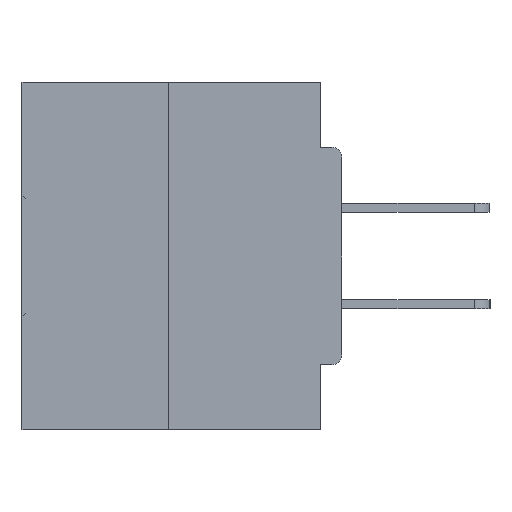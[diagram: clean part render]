
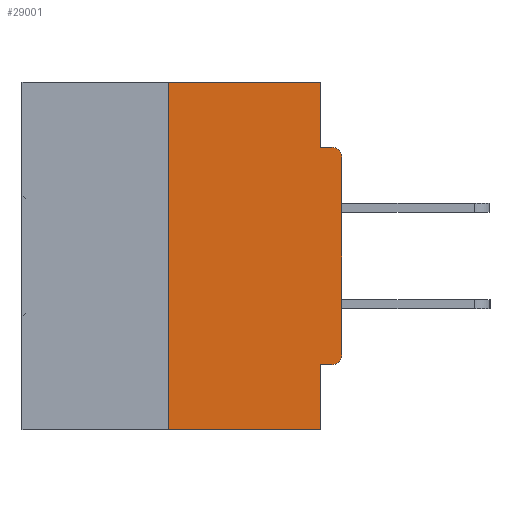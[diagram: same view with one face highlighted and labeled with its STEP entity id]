
A CAD part, left-side view. The second image highlights one B-rep face of the part: STEP entity #29001.
In plain terms, the highlighted planar face has unit normal (-1, 0, 0).
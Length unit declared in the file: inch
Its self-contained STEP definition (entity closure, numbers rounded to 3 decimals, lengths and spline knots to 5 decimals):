
#209 = CARTESIAN_POINT ( 'NONE',  ( 0., 0., -0.4065 ) ) ;
#803 = DIRECTION ( 'NONE',  ( 0., -1., 0. ) ) ;
#871 = VECTOR ( 'NONE', #2284, 39.37008 ) ;
#1094 = CARTESIAN_POINT ( 'NONE',  ( 0., 0.015, -0.4065 ) ) ;
#1310 = DIRECTION ( 'NONE',  ( 0., 0., -1. ) ) ;
#2025 = VERTEX_POINT ( 'NONE', #38893 ) ;
#2284 = DIRECTION ( 'NONE',  ( 0., 0., -1. ) ) ;
#2724 = DIRECTION ( 'NONE',  ( -1., 0., 0. ) ) ;
#3102 = CARTESIAN_POINT ( 'NONE',  ( 0., 0., -0.1085 ) ) ;
#3535 = CARTESIAN_POINT ( 'NONE',  ( 0., 0.25, 0. ) ) ;
#3756 = EDGE_CURVE ( 'NONE', #33073, #25806, #28553, .T. ) ;
#5375 = EDGE_CURVE ( 'NONE', #2025, #14541, #27541, .T. ) ;
#5636 = ORIENTED_EDGE ( 'NONE', *, *, #16228, .T. ) ;
#5768 = CARTESIAN_POINT ( 'NONE',  ( 0., 0.015, -0.3915 ) ) ;
#6494 = ORIENTED_EDGE ( 'NONE', *, *, #5375, .F. ) ;
#9302 = VECTOR ( 'NONE', #24509, 39.37008 ) ;
#9380 = ORIENTED_EDGE ( 'NONE', *, *, #10526, .T. ) ;
#9419 = VERTEX_POINT ( 'NONE', #3102 ) ;
#10275 = CARTESIAN_POINT ( 'NONE',  ( 0., 0.46, -0.5 ) ) ;
#10526 = EDGE_CURVE ( 'NONE', #12699, #25806, #32915, .T. ) ;
#11445 = EDGE_CURVE ( 'NONE', #33711, #33073, #29944, .T. ) ;
#12699 = VERTEX_POINT ( 'NONE', #19919 ) ;
#12700 = EDGE_LOOP ( 'NONE', ( #19458, #32668, #9380, #21353, #15758, #39496, #5636, #24989, #30597, #6494 ) ) ;
#12721 = VECTOR ( 'NONE', #803, 39.37008 ) ;
#14541 = VERTEX_POINT ( 'NONE', #25181 ) ;
#14918 = VECTOR ( 'NONE', #36881, 39.37008 ) ;
#15758 = ORIENTED_EDGE ( 'NONE', *, *, #11445, .F. ) ;
#15767 = DIRECTION ( 'NONE',  ( 0., -1., 0. ) ) ;
#16208 = LINE ( 'NONE', #32558, #35334 ) ;
#16228 = EDGE_CURVE ( 'NONE', #28653, #9419, #24288, .T. ) ;
#17284 = CARTESIAN_POINT ( 'NONE',  ( 0., 0., -0.0935 ) ) ;
#17497 = LINE ( 'NONE', #17284, #12721 ) ;
#19458 = ORIENTED_EDGE ( 'NONE', *, *, #29046, .F. ) ;
#19919 = CARTESIAN_POINT ( 'NONE',  ( 0., 0.25, -0.5 ) ) ;
#20221 = AXIS2_PLACEMENT_3D ( 'NONE', #5768, #28376, #38171 ) ;
#21062 = CARTESIAN_POINT ( 'NONE',  ( 0., 0.46, 0. ) ) ;
#21353 = ORIENTED_EDGE ( 'NONE', *, *, #3756, .F. ) ;
#22382 = CARTESIAN_POINT ( 'NONE',  ( 0., 0., -0.3915 ) ) ;
#23058 = CIRCLE ( 'NONE', #32781, 0.015 ) ;
#23526 = DIRECTION ( 'NONE',  ( 0., -1., 0. ) ) ;
#23852 = CARTESIAN_POINT ( 'NONE',  ( 0., 0.031, 0. ) ) ;
#24288 = LINE ( 'NONE', #31470, #37055 ) ;
#24320 = PLANE ( 'NONE',  #31164 ) ;
#24509 = DIRECTION ( 'NONE',  ( 0., 0., -1. ) ) ;
#24989 = ORIENTED_EDGE ( 'NONE', *, *, #27829, .T. ) ;
#25181 = CARTESIAN_POINT ( 'NONE',  ( 0., 0.031, -0.0935 ) ) ;
#25806 = VERTEX_POINT ( 'NONE', #35751 ) ;
#27541 = LINE ( 'NONE', #23852, #9302 ) ;
#27630 = EDGE_CURVE ( 'NONE', #33711, #28653, #35540, .T. ) ;
#27829 = EDGE_CURVE ( 'NONE', #9419, #33159, #23058, .T. ) ;
#28376 = DIRECTION ( 'NONE',  ( -1., 0., 0. ) ) ;
#28553 = LINE ( 'NONE', #38150, #871 ) ;
#28653 = VERTEX_POINT ( 'NONE', #22382 ) ;
#29001 = ADVANCED_FACE ( 'NONE', ( #40858 ), #24320, .F. ) ;
#29046 = EDGE_CURVE ( 'NONE', #29495, #2025, #16208, .T. ) ;
#29182 = VECTOR ( 'NONE', #29530, 39.37008 ) ;
#29495 = VERTEX_POINT ( 'NONE', #3535 ) ;
#29530 = DIRECTION ( 'NONE',  ( 0., 1., 0. ) ) ;
#29600 = CARTESIAN_POINT ( 'NONE',  ( 0., 0.015, -0.0935 ) ) ;
#29944 = LINE ( 'NONE', #209, #29182 ) ;
#30597 = ORIENTED_EDGE ( 'NONE', *, *, #38209, .F. ) ;
#31078 = DIRECTION ( 'NONE',  ( 1., 0., 0. ) ) ;
#31164 = AXIS2_PLACEMENT_3D ( 'NONE', #21062, #31078, #1310 ) ;
#31470 = CARTESIAN_POINT ( 'NONE',  ( 0., 0., 0. ) ) ;
#32558 = CARTESIAN_POINT ( 'NONE',  ( 0., 0.46, 0. ) ) ;
#32668 = ORIENTED_EDGE ( 'NONE', *, *, #39511, .F. ) ;
#32781 = AXIS2_PLACEMENT_3D ( 'NONE', #33363, #2724, #39014 ) ;
#32915 = LINE ( 'NONE', #10275, #36178 ) ;
#33073 = VERTEX_POINT ( 'NONE', #37955 ) ;
#33159 = VERTEX_POINT ( 'NONE', #29600 ) ;
#33363 = CARTESIAN_POINT ( 'NONE',  ( 0., 0.015, -0.1085 ) ) ;
#33416 = LINE ( 'NONE', #33855, #14918 ) ;
#33711 = VERTEX_POINT ( 'NONE', #1094 ) ;
#33855 = CARTESIAN_POINT ( 'NONE',  ( 0., 0.25, 0. ) ) ;
#35334 = VECTOR ( 'NONE', #15767, 39.37008 ) ;
#35540 = CIRCLE ( 'NONE', #20221, 0.015 ) ;
#35751 = CARTESIAN_POINT ( 'NONE',  ( 0., 0.031, -0.5 ) ) ;
#36178 = VECTOR ( 'NONE', #23526, 39.37008 ) ;
#36881 = DIRECTION ( 'NONE',  ( 0., 0., 1. ) ) ;
#37055 = VECTOR ( 'NONE', #41242, 39.37008 ) ;
#37955 = CARTESIAN_POINT ( 'NONE',  ( 0., 0.031, -0.4065 ) ) ;
#38150 = CARTESIAN_POINT ( 'NONE',  ( 0., 0.031, -0.5 ) ) ;
#38171 = DIRECTION ( 'NONE',  ( 0., 0., -1. ) ) ;
#38209 = EDGE_CURVE ( 'NONE', #14541, #33159, #17497, .T. ) ;
#38893 = CARTESIAN_POINT ( 'NONE',  ( 0., 0.031, 0. ) ) ;
#39014 = DIRECTION ( 'NONE',  ( 0., 0., -1. ) ) ;
#39496 = ORIENTED_EDGE ( 'NONE', *, *, #27630, .T. ) ;
#39511 = EDGE_CURVE ( 'NONE', #12699, #29495, #33416, .T. ) ;
#40858 = FACE_OUTER_BOUND ( 'NONE', #12700, .T. ) ;
#41242 = DIRECTION ( 'NONE',  ( 0., 0., 1. ) ) ;
